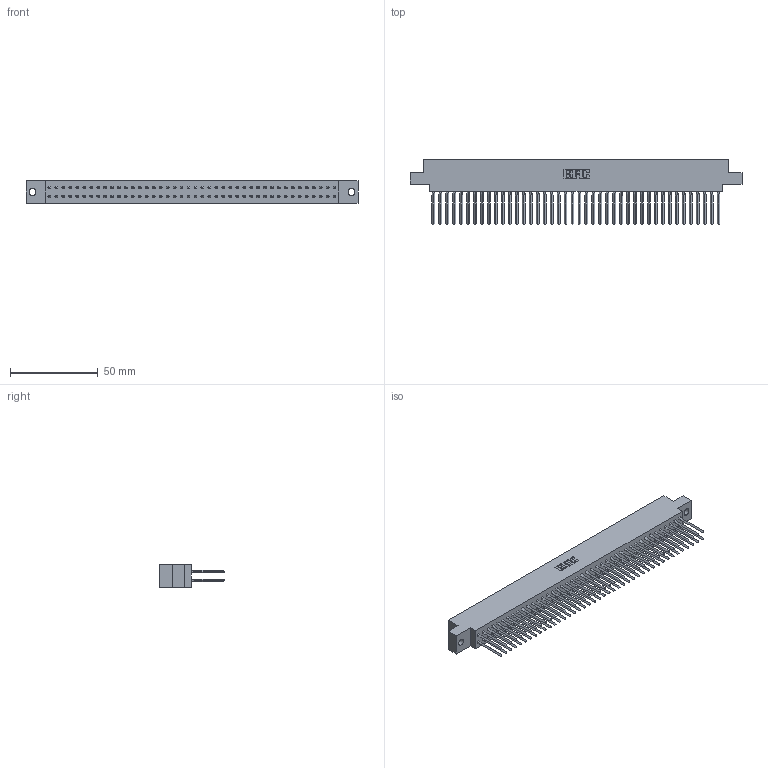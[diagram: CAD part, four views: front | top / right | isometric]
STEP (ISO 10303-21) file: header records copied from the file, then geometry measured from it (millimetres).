
FILE_DESCRIPTION (( 'STEP AP203' ), '1' );
FILE_NAME ('317-084-540-804.STEP', '2020-02-28T10:01:26', ( '' ), ( '' ), 'SwSTEP 2.0', 'SolidWorks 2016', '' );
FILE_SCHEMA (( 'CONFIG_CONTROL_DESIGN' ));
Length unit declared in the file: inch
Products named in the file (3): 317-084-540-804; 317-290-001_540; 317 Part_.156 Dia - TH
Assembly tree (85 placements, depth 2):
  317-084-540-804
    317 Part_.156 Dia - TH
    317-290-001_540  x84
Bounding box: 189.13 x 37.34 x 12.7 mm (x, y, z)
Volume: 31653.8 mm3; surface area: 47018.1 mm2
Topology: 85 solids, 85 shells, 7578 faces, 21023 edges, 13538 vertices
Faces by surface type: plane 6190, cylinder 1052, bspline 336
Entity records: 60714 total; most frequent: CARTESIAN_POINT 11007, ORIENTED_EDGE 10506, DIRECTION 8763, EDGE_CURVE 5253, VECTOR 4997, LINE 4997, VERTEX_POINT 3495, AXIS2_PLACEMENT_3D 1883
